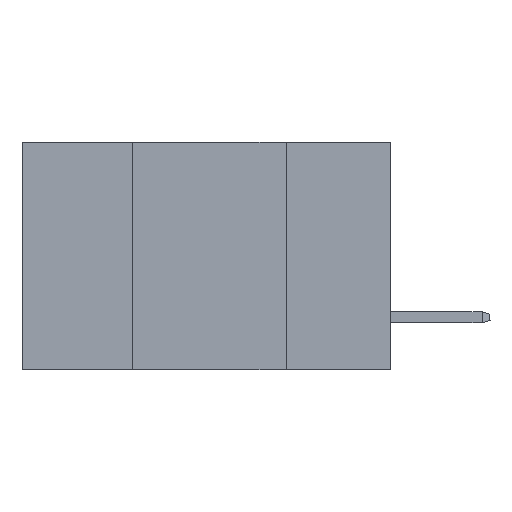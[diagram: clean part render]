
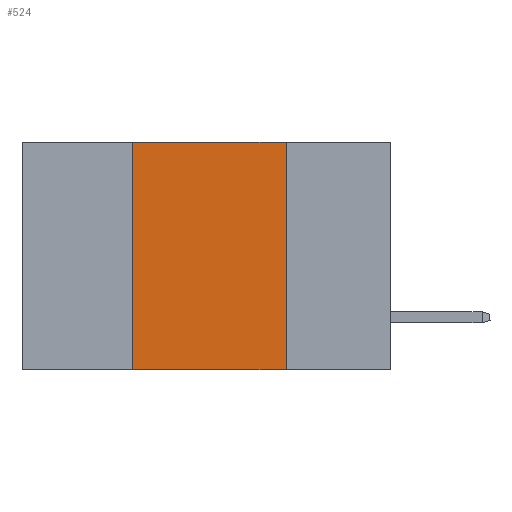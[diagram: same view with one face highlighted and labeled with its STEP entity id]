
A CAD part, left-side view. The second image highlights one B-rep face of the part: STEP entity #524.
In plain terms, the highlighted planar face has unit normal (-1, 0, 0).
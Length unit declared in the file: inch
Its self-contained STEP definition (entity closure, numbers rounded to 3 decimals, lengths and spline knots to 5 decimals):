
#212 = CARTESIAN_POINT ( 'NONE',  ( 0., 0.17, 0. ) ) ;
#524 = ADVANCED_FACE ( 'NONE', ( #16287 ), #9954, .F. ) ;
#657 = EDGE_CURVE ( 'NONE', #7077, #12210, #15352, .T. ) ;
#836 = CARTESIAN_POINT ( 'NONE',  ( 0., 0.17, 0. ) ) ;
#2153 = DIRECTION ( 'NONE',  ( 0., 0., -1. ) ) ;
#2441 = CARTESIAN_POINT ( 'NONE',  ( 0., 0.17, -0.37 ) ) ;
#2885 = AXIS2_PLACEMENT_3D ( 'NONE', #11496, #8436, #9891 ) ;
#3974 = LINE ( 'NONE', #8464, #12603 ) ;
#4949 = VECTOR ( 'NONE', #2153, 39.37008 ) ;
#5175 = LINE ( 'NONE', #836, #4949 ) ;
#5474 = EDGE_CURVE ( 'NONE', #16627, #15213, #12765, .T. ) ;
#5599 = CARTESIAN_POINT ( 'NONE',  ( 0., 0.42, 0. ) ) ;
#7077 = VERTEX_POINT ( 'NONE', #5599 ) ;
#7459 = ORIENTED_EDGE ( 'NONE', *, *, #5474, .T. ) ;
#8261 = ORIENTED_EDGE ( 'NONE', *, *, #16370, .F. ) ;
#8436 = DIRECTION ( 'NONE',  ( 1., 0., 0. ) ) ;
#8464 = CARTESIAN_POINT ( 'NONE',  ( 0., 0.42, 0. ) ) ;
#8886 = CARTESIAN_POINT ( 'NONE',  ( 0., 0.42, -0.37 ) ) ;
#9517 = ORIENTED_EDGE ( 'NONE', *, *, #657, .F. ) ;
#9742 = VECTOR ( 'NONE', #19467, 39.37008 ) ;
#9891 = DIRECTION ( 'NONE',  ( 0., 0., -1. ) ) ;
#9954 = PLANE ( 'NONE',  #2885 ) ;
#10207 = CARTESIAN_POINT ( 'NONE',  ( 0., 0.6, 0. ) ) ;
#10711 = EDGE_LOOP ( 'NONE', ( #11111, #9517, #8261, #7459 ) ) ;
#11111 = ORIENTED_EDGE ( 'NONE', *, *, #15596, .F. ) ;
#11496 = CARTESIAN_POINT ( 'NONE',  ( 0., 0.6, 0. ) ) ;
#12210 = VERTEX_POINT ( 'NONE', #212 ) ;
#12603 = VECTOR ( 'NONE', #13118, 39.37008 ) ;
#12765 = LINE ( 'NONE', #16728, #15786 ) ;
#13118 = DIRECTION ( 'NONE',  ( 0., 0., 1. ) ) ;
#15213 = VERTEX_POINT ( 'NONE', #2441 ) ;
#15352 = LINE ( 'NONE', #10207, #9742 ) ;
#15596 = EDGE_CURVE ( 'NONE', #12210, #15213, #5175, .T. ) ;
#15786 = VECTOR ( 'NONE', #18396, 39.37008 ) ;
#16287 = FACE_OUTER_BOUND ( 'NONE', #10711, .T. ) ;
#16370 = EDGE_CURVE ( 'NONE', #16627, #7077, #3974, .T. ) ;
#16627 = VERTEX_POINT ( 'NONE', #8886 ) ;
#16728 = CARTESIAN_POINT ( 'NONE',  ( 0., 0.6, -0.37 ) ) ;
#18396 = DIRECTION ( 'NONE',  ( 0., -1., 0. ) ) ;
#19467 = DIRECTION ( 'NONE',  ( 0., -1., 0. ) ) ;
